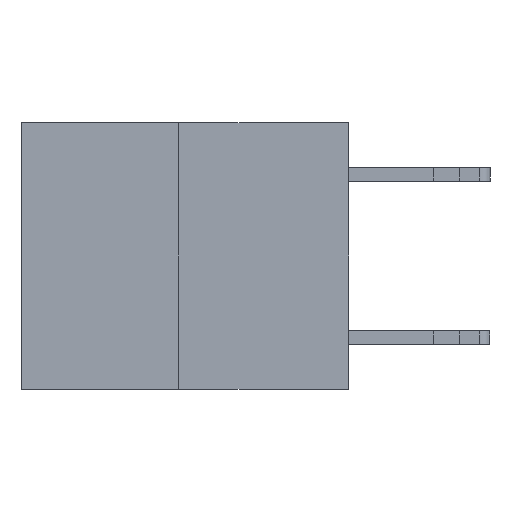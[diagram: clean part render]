
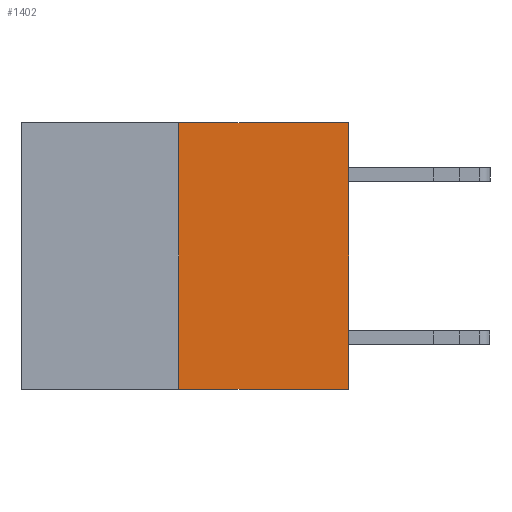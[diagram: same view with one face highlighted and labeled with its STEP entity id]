
A CAD part, left-side view. The second image highlights one B-rep face of the part: STEP entity #1402.
In plain terms, the highlighted planar face has unit normal (-1, 0, 0).
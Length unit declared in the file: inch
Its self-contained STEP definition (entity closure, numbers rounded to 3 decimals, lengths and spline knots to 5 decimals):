
#350 = DIRECTION ( 'NONE',  ( 0., -1., 0. ) ) ;
#788 = EDGE_CURVE ( 'NONE', #14674, #3433, #15573, .T. ) ;
#933 = PLANE ( 'NONE',  #7878 ) ;
#1402 = ADVANCED_FACE ( 'NONE', ( #14574 ), #933, .F. ) ;
#2184 = CARTESIAN_POINT ( 'NONE',  ( 0., 0., 0. ) ) ;
#2286 = DIRECTION ( 'NONE',  ( 1., 0., 0. ) ) ;
#2671 = LINE ( 'NONE', #14420, #15067 ) ;
#3115 = LINE ( 'NONE', #9577, #13374 ) ;
#3211 = EDGE_CURVE ( 'NONE', #14674, #16218, #12279, .T. ) ;
#3395 = DIRECTION ( 'NONE',  ( 0., 0., 1. ) ) ;
#3433 = VERTEX_POINT ( 'NONE', #15809 ) ;
#3846 = CARTESIAN_POINT ( 'NONE',  ( 0., 0.312, -0.49 ) ) ;
#5655 = DIRECTION ( 'NONE',  ( 0., -1., 0. ) ) ;
#6486 = EDGE_CURVE ( 'NONE', #16218, #13959, #3115, .T. ) ;
#7878 = AXIS2_PLACEMENT_3D ( 'NONE', #8562, #2286, #16140 ) ;
#8562 = CARTESIAN_POINT ( 'NONE',  ( 0., 0.6, 0. ) ) ;
#9189 = ORIENTED_EDGE ( 'NONE', *, *, #6486, .T. ) ;
#9577 = CARTESIAN_POINT ( 'NONE',  ( 0., 0., 0. ) ) ;
#9871 = VECTOR ( 'NONE', #10894, 39.37008 ) ;
#9905 = ORIENTED_EDGE ( 'NONE', *, *, #3211, .T. ) ;
#10513 = VECTOR ( 'NONE', #5655, 39.37008 ) ;
#10894 = DIRECTION ( 'NONE',  ( 0., 0., 1. ) ) ;
#11372 = ORIENTED_EDGE ( 'NONE', *, *, #13553, .F. ) ;
#11928 = CARTESIAN_POINT ( 'NONE',  ( 0., 0.6, -0.49 ) ) ;
#12279 = LINE ( 'NONE', #11928, #10513 ) ;
#12475 = CARTESIAN_POINT ( 'NONE',  ( 0., 0., -0.49 ) ) ;
#13277 = EDGE_LOOP ( 'NONE', ( #13373, #9905, #9189, #11372 ) ) ;
#13373 = ORIENTED_EDGE ( 'NONE', *, *, #788, .F. ) ;
#13374 = VECTOR ( 'NONE', #3395, 39.37008 ) ;
#13553 = EDGE_CURVE ( 'NONE', #3433, #13959, #2671, .T. ) ;
#13959 = VERTEX_POINT ( 'NONE', #2184 ) ;
#14420 = CARTESIAN_POINT ( 'NONE',  ( 0., 0.6, 0. ) ) ;
#14574 = FACE_OUTER_BOUND ( 'NONE', #13277, .T. ) ;
#14674 = VERTEX_POINT ( 'NONE', #3846 ) ;
#15067 = VECTOR ( 'NONE', #350, 39.37008 ) ;
#15573 = LINE ( 'NONE', #15986, #9871 ) ;
#15809 = CARTESIAN_POINT ( 'NONE',  ( 0., 0.312, 0. ) ) ;
#15986 = CARTESIAN_POINT ( 'NONE',  ( 0., 0.312, -0.49 ) ) ;
#16140 = DIRECTION ( 'NONE',  ( 0., 0., -1. ) ) ;
#16218 = VERTEX_POINT ( 'NONE', #12475 ) ;
